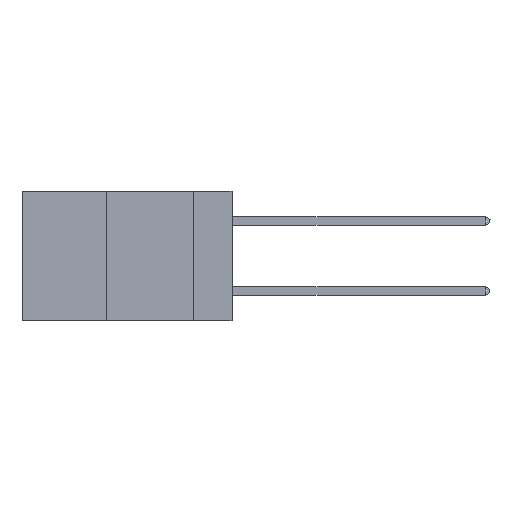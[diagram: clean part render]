
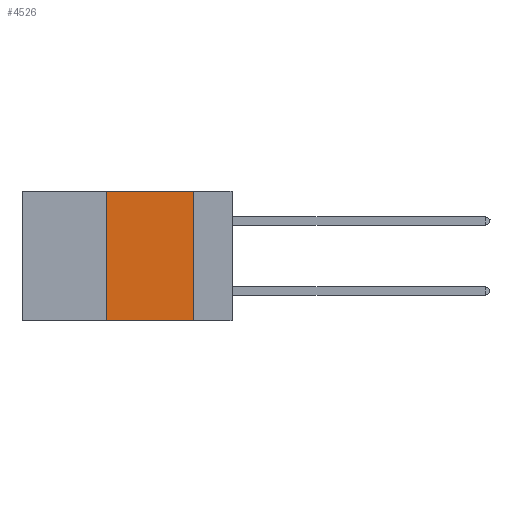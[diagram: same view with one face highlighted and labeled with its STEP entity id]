
A CAD part, left-side view. The second image highlights one B-rep face of the part: STEP entity #4526.
In plain terms, the highlighted planar face has unit normal (-1, 0, 0).
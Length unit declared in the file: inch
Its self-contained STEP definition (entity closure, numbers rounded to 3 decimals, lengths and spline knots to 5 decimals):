
#149 = VERTEX_POINT ( 'NONE', #3646 ) ;
#598 = CARTESIAN_POINT ( 'NONE',  ( 0., 0.11, 0. ) ) ;
#726 = LINE ( 'NONE', #598, #8874 ) ;
#896 = CARTESIAN_POINT ( 'NONE',  ( 0., 0.6, -0.37 ) ) ;
#1103 = LINE ( 'NONE', #896, #2282 ) ;
#1442 = DIRECTION ( 'NONE',  ( 1., 0., 0. ) ) ;
#1729 = CARTESIAN_POINT ( 'NONE',  ( 0., 0.36, 0. ) ) ;
#2282 = VECTOR ( 'NONE', #5230, 39.37008 ) ;
#2457 = ORIENTED_EDGE ( 'NONE', *, *, #7918, .F. ) ;
#2732 = CARTESIAN_POINT ( 'NONE',  ( 0., 0.36, 0. ) ) ;
#3412 = CARTESIAN_POINT ( 'NONE',  ( 0., 0.11, -0.37 ) ) ;
#3646 = CARTESIAN_POINT ( 'NONE',  ( 0., 0.11, 0. ) ) ;
#3890 = ORIENTED_EDGE ( 'NONE', *, *, #10288, .F. ) ;
#3990 = DIRECTION ( 'NONE',  ( 0., -1., 0. ) ) ;
#4129 = LINE ( 'NONE', #11295, #4661 ) ;
#4526 = ADVANCED_FACE ( 'NONE', ( #5499 ), #8465, .F. ) ;
#4548 = VERTEX_POINT ( 'NONE', #2732 ) ;
#4661 = VECTOR ( 'NONE', #3990, 39.37008 ) ;
#4875 = VERTEX_POINT ( 'NONE', #3412 ) ;
#5230 = DIRECTION ( 'NONE',  ( 0., -1., 0. ) ) ;
#5499 = FACE_OUTER_BOUND ( 'NONE', #11641, .T. ) ;
#5570 = DIRECTION ( 'NONE',  ( 0., 0., -1. ) ) ;
#5589 = EDGE_CURVE ( 'NONE', #10503, #4875, #1103, .T. ) ;
#5916 = DIRECTION ( 'NONE',  ( 0., 0., -1. ) ) ;
#6212 = ORIENTED_EDGE ( 'NONE', *, *, #5589, .T. ) ;
#6352 = AXIS2_PLACEMENT_3D ( 'NONE', #10716, #1442, #5570 ) ;
#6846 = CARTESIAN_POINT ( 'NONE',  ( 0., 0.36, -0.37 ) ) ;
#7867 = VECTOR ( 'NONE', #11007, 39.37008 ) ;
#7918 = EDGE_CURVE ( 'NONE', #10503, #4548, #8891, .T. ) ;
#8465 = PLANE ( 'NONE',  #6352 ) ;
#8771 = EDGE_CURVE ( 'NONE', #149, #4875, #726, .T. ) ;
#8874 = VECTOR ( 'NONE', #5916, 39.37008 ) ;
#8891 = LINE ( 'NONE', #1729, #7867 ) ;
#10288 = EDGE_CURVE ( 'NONE', #4548, #149, #4129, .T. ) ;
#10503 = VERTEX_POINT ( 'NONE', #6846 ) ;
#10716 = CARTESIAN_POINT ( 'NONE',  ( 0., 0.6, 0. ) ) ;
#11007 = DIRECTION ( 'NONE',  ( 0., 0., 1. ) ) ;
#11295 = CARTESIAN_POINT ( 'NONE',  ( 0., 0.6, 0. ) ) ;
#11641 = EDGE_LOOP ( 'NONE', ( #12351, #3890, #2457, #6212 ) ) ;
#12351 = ORIENTED_EDGE ( 'NONE', *, *, #8771, .F. ) ;
